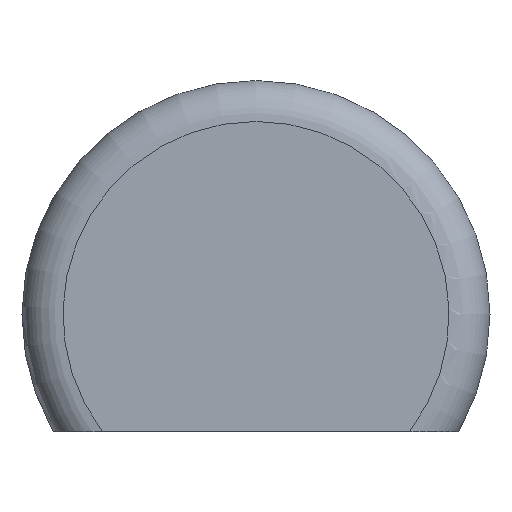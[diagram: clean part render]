
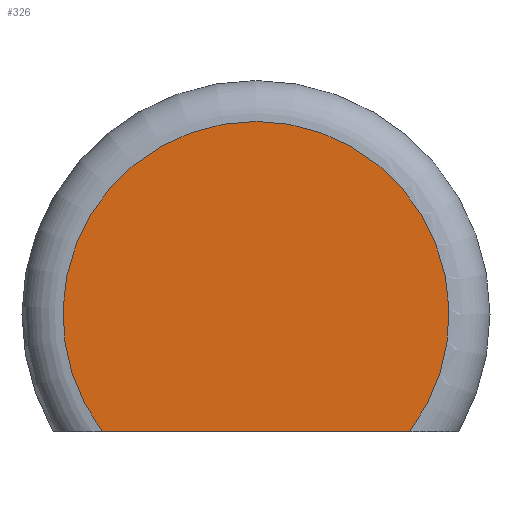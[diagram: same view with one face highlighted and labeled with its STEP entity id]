
A CAD part, front view. The second image highlights one B-rep face of the part: STEP entity #326.
In plain terms, the highlighted planar face has unit normal (0, -1, 0).
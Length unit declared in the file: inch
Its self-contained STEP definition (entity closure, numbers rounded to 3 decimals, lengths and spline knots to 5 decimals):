
#2 = EDGE_CURVE ( 'NONE', #32, #143, #328, .T. ) ;
#32 = VERTEX_POINT ( 'NONE', #206 ) ;
#43 = CARTESIAN_POINT ( 'NONE',  ( 0.13124, -0.05906, -0.1 ) ) ;
#61 = DIRECTION ( 'NONE',  ( 0., 0., -1. ) ) ;
#74 = DIRECTION ( 'NONE',  ( 1., 0., 0. ) ) ;
#91 = CARTESIAN_POINT ( 'NONE',  ( 0., -0.05906, 0. ) ) ;
#112 = EDGE_CURVE ( 'NONE', #143, #32, #393, .T. ) ;
#123 = ORIENTED_EDGE ( 'NONE', *, *, #112, .T. ) ;
#138 = CARTESIAN_POINT ( 'NONE',  ( 0., -0.05906, 0. ) ) ;
#143 = VERTEX_POINT ( 'NONE', #43 ) ;
#162 = ORIENTED_EDGE ( 'NONE', *, *, #2, .T. ) ;
#199 = CARTESIAN_POINT ( 'NONE',  ( 0.17321, -0.05906, -0.1 ) ) ;
#203 = AXIS2_PLACEMENT_3D ( 'NONE', #91, #386, #61 ) ;
#204 = DIRECTION ( 'NONE',  ( 0., -1., 0. ) ) ;
#206 = CARTESIAN_POINT ( 'NONE',  ( -0.13124, -0.05906, -0.1 ) ) ;
#238 = EDGE_LOOP ( 'NONE', ( #162, #123 ) ) ;
#255 = PLANE ( 'NONE',  #203 ) ;
#308 = DIRECTION ( 'NONE',  ( 0., 0., -1. ) ) ;
#326 = ADVANCED_FACE ( 'NONE', ( #366 ), #255, .T. ) ;
#328 = LINE ( 'NONE', #199, #394 ) ;
#366 = FACE_OUTER_BOUND ( 'NONE', #238, .T. ) ;
#367 = AXIS2_PLACEMENT_3D ( 'NONE', #138, #204, #308 ) ;
#386 = DIRECTION ( 'NONE',  ( 0., -1., 0. ) ) ;
#393 = CIRCLE ( 'NONE', #367, 0.165 ) ;
#394 = VECTOR ( 'NONE', #74, 39.37008 ) ;
